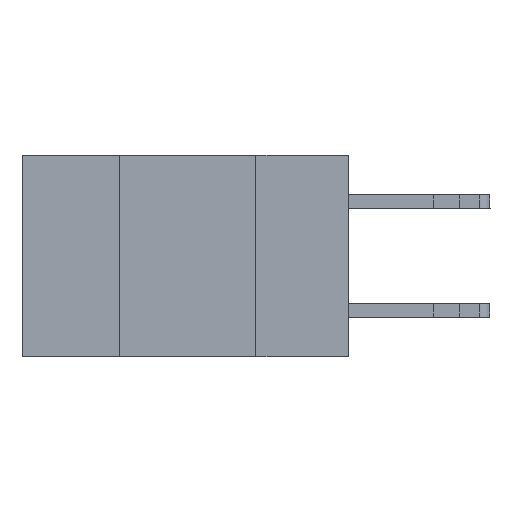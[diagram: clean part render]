
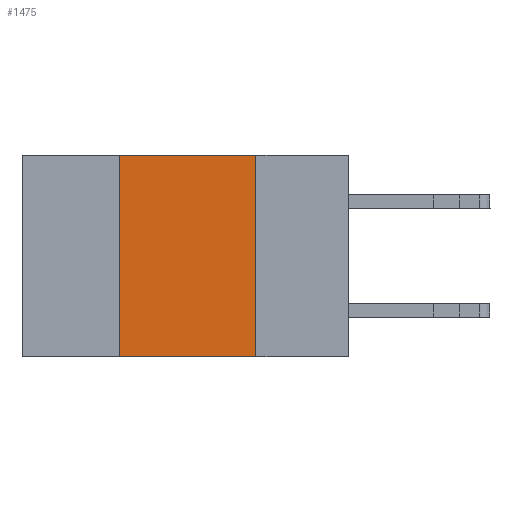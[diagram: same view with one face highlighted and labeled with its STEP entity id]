
A CAD part, left-side view. The second image highlights one B-rep face of the part: STEP entity #1475.
In plain terms, the highlighted planar face has unit normal (-1, 0, 0).
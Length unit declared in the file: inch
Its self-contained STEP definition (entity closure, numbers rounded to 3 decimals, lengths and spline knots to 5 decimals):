
#482 = EDGE_CURVE ( 'NONE', #1386, #5620, #8015, .T. ) ;
#696 = CARTESIAN_POINT ( 'NONE',  ( 0., 0.42, 0. ) ) ;
#905 = CARTESIAN_POINT ( 'NONE',  ( 0., 0.42, -0.37 ) ) ;
#950 = CARTESIAN_POINT ( 'NONE',  ( 0., 0.17, 0. ) ) ;
#1273 = DIRECTION ( 'NONE',  ( 1., 0., 0. ) ) ;
#1297 = VECTOR ( 'NONE', #2997, 39.37008 ) ;
#1345 = CARTESIAN_POINT ( 'NONE',  ( 0., 0.17, -0.37 ) ) ;
#1386 = VERTEX_POINT ( 'NONE', #950 ) ;
#1475 = ADVANCED_FACE ( 'NONE', ( #2125 ), #7220, .F. ) ;
#2076 = CARTESIAN_POINT ( 'NONE',  ( 0., 0.6, 0. ) ) ;
#2125 = FACE_OUTER_BOUND ( 'NONE', #6367, .T. ) ;
#2278 = VERTEX_POINT ( 'NONE', #905 ) ;
#2640 = ORIENTED_EDGE ( 'NONE', *, *, #482, .F. ) ;
#2885 = CARTESIAN_POINT ( 'NONE',  ( 0., 0.17, -0.37 ) ) ;
#2997 = DIRECTION ( 'NONE',  ( 0., 0., 1. ) ) ;
#3047 = CARTESIAN_POINT ( 'NONE',  ( 0., 0.42, -0.37 ) ) ;
#3066 = VECTOR ( 'NONE', #3425, 39.37008 ) ;
#3425 = DIRECTION ( 'NONE',  ( 0., -1., 0. ) ) ;
#4529 = EDGE_CURVE ( 'NONE', #2278, #5620, #6941, .T. ) ;
#4566 = DIRECTION ( 'NONE',  ( 0., 0., -1. ) ) ;
#4792 = DIRECTION ( 'NONE',  ( 0., 0., -1. ) ) ;
#4919 = LINE ( 'NONE', #3047, #1297 ) ;
#5013 = ORIENTED_EDGE ( 'NONE', *, *, #8042, .F. ) ;
#5570 = ORIENTED_EDGE ( 'NONE', *, *, #4529, .T. ) ;
#5620 = VERTEX_POINT ( 'NONE', #2885 ) ;
#6367 = EDGE_LOOP ( 'NONE', ( #2640, #5013, #6490, #5570 ) ) ;
#6490 = ORIENTED_EDGE ( 'NONE', *, *, #7002, .F. ) ;
#6702 = AXIS2_PLACEMENT_3D ( 'NONE', #2076, #1273, #4566 ) ;
#6941 = LINE ( 'NONE', #9575, #3066 ) ;
#7002 = EDGE_CURVE ( 'NONE', #2278, #10493, #4919, .T. ) ;
#7220 = PLANE ( 'NONE',  #6702 ) ;
#7809 = DIRECTION ( 'NONE',  ( 0., -1., 0. ) ) ;
#8015 = LINE ( 'NONE', #1345, #8725 ) ;
#8042 = EDGE_CURVE ( 'NONE', #10493, #1386, #8589, .T. ) ;
#8589 = LINE ( 'NONE', #8712, #9255 ) ;
#8712 = CARTESIAN_POINT ( 'NONE',  ( 0., 0.6, 0. ) ) ;
#8725 = VECTOR ( 'NONE', #4792, 39.37008 ) ;
#9255 = VECTOR ( 'NONE', #7809, 39.37008 ) ;
#9575 = CARTESIAN_POINT ( 'NONE',  ( 0., 0.6, -0.37 ) ) ;
#10493 = VERTEX_POINT ( 'NONE', #696 ) ;
